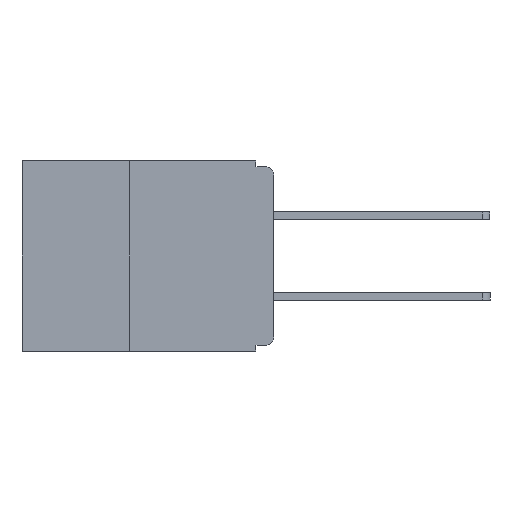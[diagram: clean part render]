
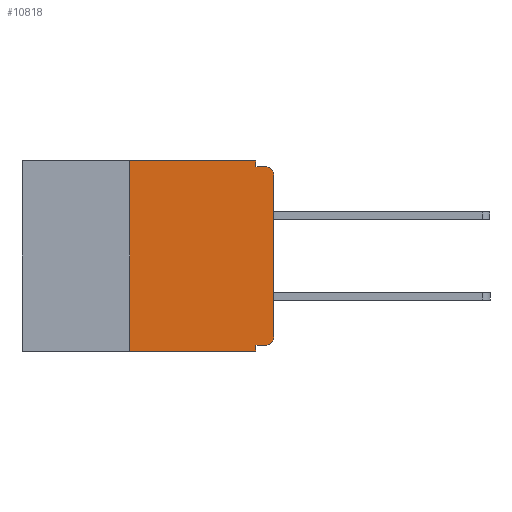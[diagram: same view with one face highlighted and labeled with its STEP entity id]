
A CAD part, left-side view. The second image highlights one B-rep face of the part: STEP entity #10818.
In plain terms, the highlighted planar face has unit normal (-1, 0, 0).
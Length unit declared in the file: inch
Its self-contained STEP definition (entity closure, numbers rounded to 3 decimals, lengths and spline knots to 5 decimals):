
#219 = DIRECTION ( 'NONE',  ( 1., 0., 0. ) ) ;
#257 = CARTESIAN_POINT ( 'NONE',  ( 0., 0.031, -0.33 ) ) ;
#332 = DIRECTION ( 'NONE',  ( 0., 0., 1. ) ) ;
#408 = EDGE_CURVE ( 'NONE', #2787, #2994, #11452, .T. ) ;
#745 = EDGE_LOOP ( 'NONE', ( #8001, #8261, #9624, #10172, #11191, #11677, #12107, #13073, #13410, #13585 ) ) ;
#1407 = VECTOR ( 'NONE', #16126, 39.37008 ) ;
#1721 = LINE ( 'NONE', #6806, #16691 ) ;
#1982 = VERTEX_POINT ( 'NONE', #16605 ) ;
#2167 = AXIS2_PLACEMENT_3D ( 'NONE', #11838, #219, #10415 ) ;
#2291 = CARTESIAN_POINT ( 'NONE',  ( 0., 0.015, -0.305 ) ) ;
#2461 = DIRECTION ( 'NONE',  ( 0., 0., -1. ) ) ;
#2480 = VERTEX_POINT ( 'NONE', #12729 ) ;
#2685 = LINE ( 'NONE', #8759, #10458 ) ;
#2760 = CARTESIAN_POINT ( 'NONE',  ( 0., 0.015, -0.025 ) ) ;
#2787 = VERTEX_POINT ( 'NONE', #4515 ) ;
#2994 = VERTEX_POINT ( 'NONE', #16400 ) ;
#3639 = CARTESIAN_POINT ( 'NONE',  ( 0., 0.031, 0. ) ) ;
#3751 = LINE ( 'NONE', #17600, #11078 ) ;
#3763 = DIRECTION ( 'NONE',  ( 0., 0., -1. ) ) ;
#3930 = CARTESIAN_POINT ( 'NONE',  ( 0., 0.25, -0.33 ) ) ;
#4238 = DIRECTION ( 'NONE',  ( 0., 0., -1. ) ) ;
#4515 = CARTESIAN_POINT ( 'NONE',  ( 0., 0.031, -0.32 ) ) ;
#5419 = VERTEX_POINT ( 'NONE', #3639 ) ;
#5700 = LINE ( 'NONE', #17487, #1407 ) ;
#5852 = EDGE_CURVE ( 'NONE', #2480, #2994, #3751, .T. ) ;
#6015 = VERTEX_POINT ( 'NONE', #10786 ) ;
#6806 = CARTESIAN_POINT ( 'NONE',  ( 0., 0.031, 0. ) ) ;
#6941 = VERTEX_POINT ( 'NONE', #12033 ) ;
#6958 = LINE ( 'NONE', #3930, #14771 ) ;
#7764 = DIRECTION ( 'NONE',  ( 0., 0., -1. ) ) ;
#7924 = LINE ( 'NONE', #17631, #15243 ) ;
#8001 = ORIENTED_EDGE ( 'NONE', *, *, #17319, .T. ) ;
#8118 = VERTEX_POINT ( 'NONE', #13025 ) ;
#8244 = EDGE_CURVE ( 'NONE', #6015, #5419, #5700, .T. ) ;
#8261 = ORIENTED_EDGE ( 'NONE', *, *, #12964, .T. ) ;
#8759 = CARTESIAN_POINT ( 'NONE',  ( 0., 0., -0.32 ) ) ;
#8802 = CIRCLE ( 'NONE', #12732, 0.015 ) ;
#9624 = ORIENTED_EDGE ( 'NONE', *, *, #9938, .F. ) ;
#9808 = LINE ( 'NONE', #14374, #17006 ) ;
#9938 = EDGE_CURVE ( 'NONE', #1982, #11040, #9808, .T. ) ;
#10172 = ORIENTED_EDGE ( 'NONE', *, *, #14080, .F. ) ;
#10263 = AXIS2_PLACEMENT_3D ( 'NONE', #2291, #12554, #3763 ) ;
#10415 = DIRECTION ( 'NONE',  ( 0., 0., -1. ) ) ;
#10458 = VECTOR ( 'NONE', #14626, 39.37008 ) ;
#10786 = CARTESIAN_POINT ( 'NONE',  ( 0., 0.25, 0. ) ) ;
#10818 = ADVANCED_FACE ( 'NONE', ( #17842 ), #17526, .F. ) ;
#11040 = VERTEX_POINT ( 'NONE', #14553 ) ;
#11068 = EDGE_CURVE ( 'NONE', #12352, #2787, #2685, .T. ) ;
#11078 = VECTOR ( 'NONE', #17815, 39.37008 ) ;
#11191 = ORIENTED_EDGE ( 'NONE', *, *, #8244, .F. ) ;
#11452 = LINE ( 'NONE', #257, #18491 ) ;
#11677 = ORIENTED_EDGE ( 'NONE', *, *, #18248, .F. ) ;
#11838 = CARTESIAN_POINT ( 'NONE',  ( 0., 0.437, 0. ) ) ;
#12033 = CARTESIAN_POINT ( 'NONE',  ( 0., 0., -0.305 ) ) ;
#12107 = ORIENTED_EDGE ( 'NONE', *, *, #5852, .T. ) ;
#12352 = VERTEX_POINT ( 'NONE', #13040 ) ;
#12554 = DIRECTION ( 'NONE',  ( -1., 0., 0. ) ) ;
#12729 = CARTESIAN_POINT ( 'NONE',  ( 0., 0.25, -0.33 ) ) ;
#12732 = AXIS2_PLACEMENT_3D ( 'NONE', #2760, #13017, #4238 ) ;
#12964 = EDGE_CURVE ( 'NONE', #8118, #11040, #8802, .T. ) ;
#13017 = DIRECTION ( 'NONE',  ( -1., 0., 0. ) ) ;
#13025 = CARTESIAN_POINT ( 'NONE',  ( 0., 0., -0.025 ) ) ;
#13040 = CARTESIAN_POINT ( 'NONE',  ( 0., 0.015, -0.32 ) ) ;
#13073 = ORIENTED_EDGE ( 'NONE', *, *, #408, .F. ) ;
#13410 = ORIENTED_EDGE ( 'NONE', *, *, #11068, .F. ) ;
#13585 = ORIENTED_EDGE ( 'NONE', *, *, #13974, .T. ) ;
#13974 = EDGE_CURVE ( 'NONE', #12352, #6941, #14301, .T. ) ;
#14080 = EDGE_CURVE ( 'NONE', #5419, #1982, #1721, .T. ) ;
#14301 = CIRCLE ( 'NONE', #10263, 0.015 ) ;
#14374 = CARTESIAN_POINT ( 'NONE',  ( 0., 0., -0.01 ) ) ;
#14553 = CARTESIAN_POINT ( 'NONE',  ( 0., 0.015, -0.01 ) ) ;
#14626 = DIRECTION ( 'NONE',  ( 0., 1., 0. ) ) ;
#14771 = VECTOR ( 'NONE', #18256, 39.37008 ) ;
#15243 = VECTOR ( 'NONE', #332, 39.37008 ) ;
#15780 = DIRECTION ( 'NONE',  ( 0., -1., 0. ) ) ;
#16126 = DIRECTION ( 'NONE',  ( 0., -1., 0. ) ) ;
#16400 = CARTESIAN_POINT ( 'NONE',  ( 0., 0.031, -0.33 ) ) ;
#16605 = CARTESIAN_POINT ( 'NONE',  ( 0., 0.031, -0.01 ) ) ;
#16691 = VECTOR ( 'NONE', #2461, 39.37008 ) ;
#17006 = VECTOR ( 'NONE', #15780, 39.37008 ) ;
#17319 = EDGE_CURVE ( 'NONE', #6941, #8118, #7924, .T. ) ;
#17487 = CARTESIAN_POINT ( 'NONE',  ( 0., 0.437, 0. ) ) ;
#17526 = PLANE ( 'NONE',  #2167 ) ;
#17600 = CARTESIAN_POINT ( 'NONE',  ( 0., 0.437, -0.33 ) ) ;
#17631 = CARTESIAN_POINT ( 'NONE',  ( 0., 0., 0. ) ) ;
#17815 = DIRECTION ( 'NONE',  ( 0., -1., 0. ) ) ;
#17842 = FACE_OUTER_BOUND ( 'NONE', #745, .T. ) ;
#18248 = EDGE_CURVE ( 'NONE', #2480, #6015, #6958, .T. ) ;
#18256 = DIRECTION ( 'NONE',  ( 0., 0., 1. ) ) ;
#18491 = VECTOR ( 'NONE', #7764, 39.37008 ) ;
